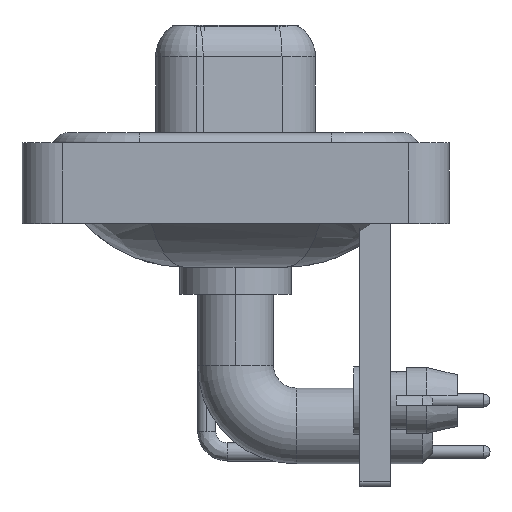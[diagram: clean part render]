
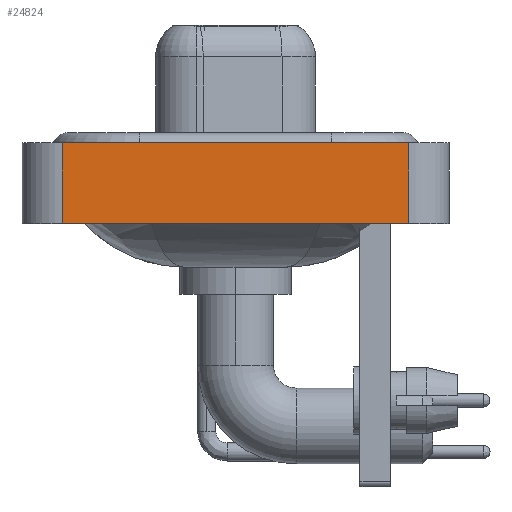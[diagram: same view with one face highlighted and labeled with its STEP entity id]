
A CAD part, left-side view. The second image highlights one B-rep face of the part: STEP entity #24824.
In plain terms, the highlighted planar face has unit normal (-1, 0, 0).
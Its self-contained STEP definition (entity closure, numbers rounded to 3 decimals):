
#1028 = CARTESIAN_POINT ( 'NONE',  ( -7.35, 8.55, -3.6 ) ) ;
#1647 = CARTESIAN_POINT ( 'NONE',  ( -7.35, 8.55, -3.6 ) ) ;
#1712 = VECTOR ( 'NONE', #22150, 1000. ) ;
#2233 = CARTESIAN_POINT ( 'NONE',  ( -7.35, -8.55, -3.6 ) ) ;
#2234 = VERTEX_POINT ( 'NONE', #12635 ) ;
#2720 = CARTESIAN_POINT ( 'NONE',  ( -7.35, -8.55, -3.6 ) ) ;
#3616 = AXIS2_PLACEMENT_3D ( 'NONE', #2233, #4023, #17721 ) ;
#4023 = DIRECTION ( 'NONE',  ( -1., 0., 0. ) ) ;
#4569 = VERTEX_POINT ( 'NONE', #7019 ) ;
#4889 = VERTEX_POINT ( 'NONE', #1647 ) ;
#6303 = LINE ( 'NONE', #11906, #15016 ) ;
#6887 = VECTOR ( 'NONE', #10510, 1000. ) ;
#7019 = CARTESIAN_POINT ( 'NONE',  ( -7.35, -8.55, 0.4 ) ) ;
#7699 = DIRECTION ( 'NONE',  ( 0., -1., 0. ) ) ;
#10112 = EDGE_CURVE ( 'NONE', #4889, #22333, #16904, .T. ) ;
#10274 = FACE_OUTER_BOUND ( 'NONE', #21063, .T. ) ;
#10510 = DIRECTION ( 'NONE',  ( 0., -1., 0. ) ) ;
#10986 = EDGE_CURVE ( 'NONE', #2234, #4569, #14607, .T. ) ;
#11116 = VECTOR ( 'NONE', #24746, 1000. ) ;
#11798 = PLANE ( 'NONE',  #3616 ) ;
#11906 = CARTESIAN_POINT ( 'NONE',  ( -7.35, -8.55, 0.4 ) ) ;
#12436 = LINE ( 'NONE', #2720, #6887 ) ;
#12543 = CARTESIAN_POINT ( 'NONE',  ( -7.35, -8.55, -3.6 ) ) ;
#12574 = ORIENTED_EDGE ( 'NONE', *, *, #10986, .T. ) ;
#12635 = CARTESIAN_POINT ( 'NONE',  ( -7.35, -8.55, -3.6 ) ) ;
#13176 = CARTESIAN_POINT ( 'NONE',  ( -7.35, 8.55, 0.4 ) ) ;
#14607 = LINE ( 'NONE', #12543, #11116 ) ;
#15016 = VECTOR ( 'NONE', #7699, 1000. ) ;
#15236 = EDGE_CURVE ( 'NONE', #22333, #4569, #6303, .T. ) ;
#15910 = ORIENTED_EDGE ( 'NONE', *, *, #10112, .F. ) ;
#16904 = LINE ( 'NONE', #1028, #1712 ) ;
#17721 = DIRECTION ( 'NONE',  ( 0., 0., 1. ) ) ;
#18301 = ORIENTED_EDGE ( 'NONE', *, *, #15236, .F. ) ;
#21063 = EDGE_LOOP ( 'NONE', ( #12574, #18301, #15910, #22720 ) ) ;
#21851 = EDGE_CURVE ( 'NONE', #4889, #2234, #12436, .T. ) ;
#22150 = DIRECTION ( 'NONE',  ( 0., 0., 1. ) ) ;
#22333 = VERTEX_POINT ( 'NONE', #13176 ) ;
#22720 = ORIENTED_EDGE ( 'NONE', *, *, #21851, .T. ) ;
#24746 = DIRECTION ( 'NONE',  ( 0., 0., 1. ) ) ;
#24824 = ADVANCED_FACE ( 'NONE', ( #10274 ), #11798, .T. ) ;
